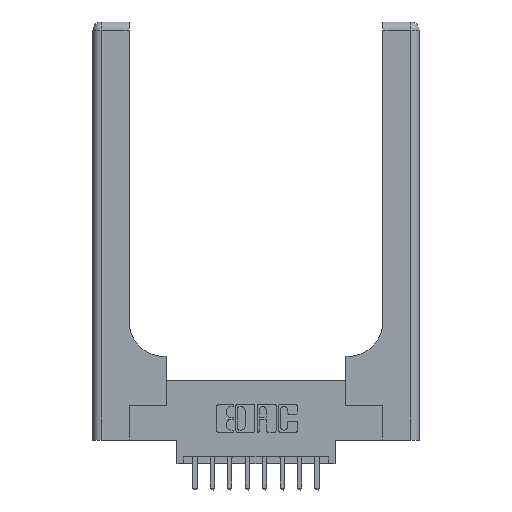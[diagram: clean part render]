
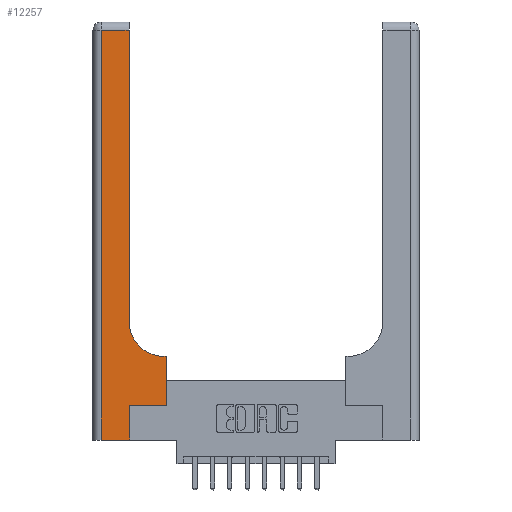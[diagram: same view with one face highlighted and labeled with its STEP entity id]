
A CAD part, top view. The second image highlights one B-rep face of the part: STEP entity #12257.
In plain terms, the highlighted planar face has unit normal (0, 0, 1).
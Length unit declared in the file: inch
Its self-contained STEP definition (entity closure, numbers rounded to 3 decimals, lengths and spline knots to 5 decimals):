
#730 = VECTOR ( 'NONE', #8104, 39.37008 ) ;
#782 = ORIENTED_EDGE ( 'NONE', *, *, #954, .T. ) ;
#954 = EDGE_CURVE ( 'NONE', #8694, #12695, #14347, .T. ) ;
#1432 = CARTESIAN_POINT ( 'NONE',  ( 0.06, 2.94, 0.37 ) ) ;
#2355 = EDGE_LOOP ( 'NONE', ( #6954, #10591, #3106, #782, #6613, #9627, #5252, #3897, #9065 ) ) ;
#2435 = CARTESIAN_POINT ( 'NONE',  ( 0.26, 0.6, 0.37 ) ) ;
#2632 = AXIS2_PLACEMENT_3D ( 'NONE', #9733, #6334, #11073 ) ;
#2971 = DIRECTION ( 'NONE',  ( 1., 0., 0. ) ) ;
#3106 = ORIENTED_EDGE ( 'NONE', *, *, #7625, .T. ) ;
#3108 = CARTESIAN_POINT ( 'NONE',  ( 0., 2.94, 0.37 ) ) ;
#3897 = ORIENTED_EDGE ( 'NONE', *, *, #4131, .T. ) ;
#4074 = LINE ( 'NONE', #9861, #14488 ) ;
#4087 = VECTOR ( 'NONE', #4154, 39.37008 ) ;
#4131 = EDGE_CURVE ( 'NONE', #11219, #10108, #13299, .T. ) ;
#4154 = DIRECTION ( 'NONE',  ( 0., 1., 0. ) ) ;
#4433 = LINE ( 'NONE', #14123, #730 ) ;
#4583 = VECTOR ( 'NONE', #13092, 39.37008 ) ;
#4609 = CARTESIAN_POINT ( 'NONE',  ( 0., 3., 0.37 ) ) ;
#4824 = EDGE_CURVE ( 'NONE', #10108, #5187, #10970, .T. ) ;
#4843 = CARTESIAN_POINT ( 'NONE',  ( 0.265, 0.25, 0.37 ) ) ;
#5187 = VERTEX_POINT ( 'NONE', #15521 ) ;
#5252 = ORIENTED_EDGE ( 'NONE', *, *, #12688, .T. ) ;
#5896 = DIRECTION ( 'NONE',  ( -1., 0., 0. ) ) ;
#6334 = DIRECTION ( 'NONE',  ( 0., 0., -1. ) ) ;
#6375 = LINE ( 'NONE', #8835, #13638 ) ;
#6469 = DIRECTION ( 'NONE',  ( 0., 1., 0. ) ) ;
#6613 = ORIENTED_EDGE ( 'NONE', *, *, #12106, .T. ) ;
#6954 = ORIENTED_EDGE ( 'NONE', *, *, #11988, .T. ) ;
#7107 = EDGE_CURVE ( 'NONE', #8334, #8428, #6375, .T. ) ;
#7625 = EDGE_CURVE ( 'NONE', #12776, #8694, #4433, .T. ) ;
#7982 = CARTESIAN_POINT ( 'NONE',  ( 0.265, 0., 0.37 ) ) ;
#8104 = DIRECTION ( 'NONE',  ( 0., -1., 0. ) ) ;
#8194 = CARTESIAN_POINT ( 'NONE',  ( 0.06, 0., 0.37 ) ) ;
#8213 = PLANE ( 'NONE',  #15266 ) ;
#8271 = CARTESIAN_POINT ( 'NONE',  ( 0.528, 0.25, 0.37 ) ) ;
#8334 = VERTEX_POINT ( 'NONE', #4843 ) ;
#8428 = VERTEX_POINT ( 'NONE', #14688 ) ;
#8694 = VERTEX_POINT ( 'NONE', #8194 ) ;
#8835 = CARTESIAN_POINT ( 'NONE',  ( 0.265, 0.25, 0.37 ) ) ;
#9049 = DIRECTION ( 'NONE',  ( -1., 0., 0. ) ) ;
#9065 = ORIENTED_EDGE ( 'NONE', *, *, #4824, .T. ) ;
#9505 = VECTOR ( 'NONE', #9049, 39.37008 ) ;
#9627 = ORIENTED_EDGE ( 'NONE', *, *, #7107, .T. ) ;
#9665 = CARTESIAN_POINT ( 'NONE',  ( 0.265, 0., 0.37 ) ) ;
#9696 = VECTOR ( 'NONE', #11048, 39.37008 ) ;
#9733 = CARTESIAN_POINT ( 'NONE',  ( 0.51, 0.85, 0.37 ) ) ;
#9861 = CARTESIAN_POINT ( 'NONE',  ( 0.26, 3., 0.37 ) ) ;
#10108 = VERTEX_POINT ( 'NONE', #10717 ) ;
#10187 = LINE ( 'NONE', #7982, #4087 ) ;
#10591 = ORIENTED_EDGE ( 'NONE', *, *, #15390, .T. ) ;
#10638 = CARTESIAN_POINT ( 'NONE',  ( 0.26, 2.94, 0.37 ) ) ;
#10717 = CARTESIAN_POINT ( 'NONE',  ( 0.51, 0.6, 0.37 ) ) ;
#10970 = CIRCLE ( 'NONE', #2632, 0.25 ) ;
#11004 = DIRECTION ( 'NONE',  ( 1., 0., 0. ) ) ;
#11048 = DIRECTION ( 'NONE',  ( -1., 0., 0. ) ) ;
#11073 = DIRECTION ( 'NONE',  ( 1., 0., 0. ) ) ;
#11219 = VERTEX_POINT ( 'NONE', #14456 ) ;
#11921 = DIRECTION ( 'NONE',  ( 0., 0., -1. ) ) ;
#11988 = EDGE_CURVE ( 'NONE', #5187, #12673, #4074, .T. ) ;
#12106 = EDGE_CURVE ( 'NONE', #12695, #8334, #10187, .T. ) ;
#12257 = ADVANCED_FACE ( 'NONE', ( #13184 ), #8213, .F. ) ;
#12673 = VERTEX_POINT ( 'NONE', #10638 ) ;
#12688 = EDGE_CURVE ( 'NONE', #8428, #11219, #14284, .T. ) ;
#12695 = VERTEX_POINT ( 'NONE', #9665 ) ;
#12776 = VERTEX_POINT ( 'NONE', #1432 ) ;
#13092 = DIRECTION ( 'NONE',  ( 0., 1., 0. ) ) ;
#13184 = FACE_OUTER_BOUND ( 'NONE', #2355, .T. ) ;
#13299 = LINE ( 'NONE', #2435, #9696 ) ;
#13638 = VECTOR ( 'NONE', #2971, 39.37008 ) ;
#13897 = LINE ( 'NONE', #3108, #9505 ) ;
#14123 = CARTESIAN_POINT ( 'NONE',  ( 0.06, 3., 0.37 ) ) ;
#14240 = VECTOR ( 'NONE', #11004, 39.37008 ) ;
#14284 = LINE ( 'NONE', #8271, #4583 ) ;
#14347 = LINE ( 'NONE', #14668, #14240 ) ;
#14456 = CARTESIAN_POINT ( 'NONE',  ( 0.528, 0.6, 0.37 ) ) ;
#14488 = VECTOR ( 'NONE', #6469, 39.37008 ) ;
#14668 = CARTESIAN_POINT ( 'NONE',  ( 0., 0., 0.37 ) ) ;
#14688 = CARTESIAN_POINT ( 'NONE',  ( 0.528, 0.25, 0.37 ) ) ;
#15266 = AXIS2_PLACEMENT_3D ( 'NONE', #4609, #11921, #5896 ) ;
#15390 = EDGE_CURVE ( 'NONE', #12673, #12776, #13897, .T. ) ;
#15521 = CARTESIAN_POINT ( 'NONE',  ( 0.26, 0.85, 0.37 ) ) ;
